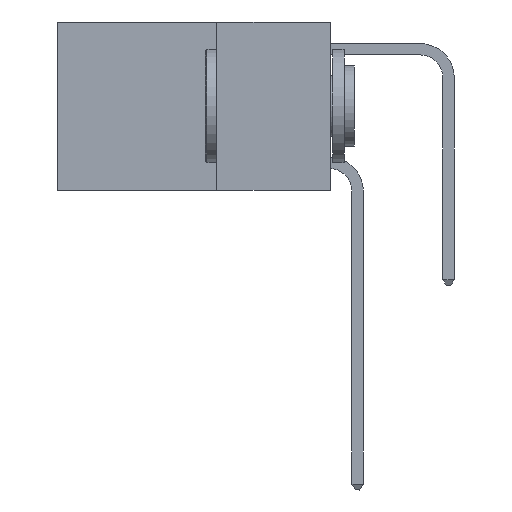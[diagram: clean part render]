
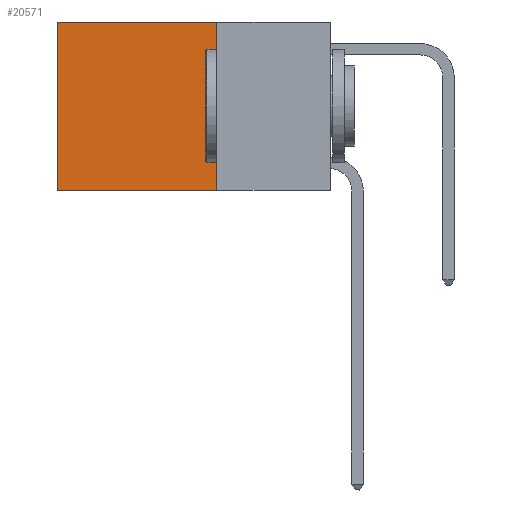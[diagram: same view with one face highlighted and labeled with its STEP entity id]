
A CAD part, left-side view. The second image highlights one B-rep face of the part: STEP entity #20571.
In plain terms, the highlighted planar face has unit normal (-1, 0, 0).
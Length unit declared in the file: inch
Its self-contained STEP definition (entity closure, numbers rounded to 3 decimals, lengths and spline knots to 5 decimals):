
#109 = CARTESIAN_POINT ( 'NONE',  ( 0.2625, 0.25, -0.37 ) ) ;
#2803 = LINE ( 'NONE', #15874, #11579 ) ;
#3349 = LINE ( 'NONE', #4680, #21914 ) ;
#3725 = VERTEX_POINT ( 'NONE', #13115 ) ;
#4546 = FACE_OUTER_BOUND ( 'NONE', #17634, .T. ) ;
#4548 = DIRECTION ( 'NONE',  ( 0., 0., -1. ) ) ;
#4680 = CARTESIAN_POINT ( 'NONE',  ( 0.2625, 0.25, 0. ) ) ;
#6588 = CARTESIAN_POINT ( 'NONE',  ( 0.2625, 0.25, 0. ) ) ;
#6670 = DIRECTION ( 'NONE',  ( 1., 0., 0. ) ) ;
#7106 = DIRECTION ( 'NONE',  ( 0., 1., 0. ) ) ;
#8659 = VECTOR ( 'NONE', #13685, 39.37008 ) ;
#8746 = ORIENTED_EDGE ( 'NONE', *, *, #20583, .T. ) ;
#9796 = VERTEX_POINT ( 'NONE', #109 ) ;
#9812 = EDGE_CURVE ( 'NONE', #9796, #16603, #2803, .T. ) ;
#9827 = CARTESIAN_POINT ( 'NONE',  ( 0.2625, 0.6, 0. ) ) ;
#10000 = VERTEX_POINT ( 'NONE', #21564 ) ;
#10196 = EDGE_CURVE ( 'NONE', #10000, #9796, #3349, .T. ) ;
#10614 = VECTOR ( 'NONE', #4548, 39.37008 ) ;
#10733 = ORIENTED_EDGE ( 'NONE', *, *, #10196, .F. ) ;
#11579 = VECTOR ( 'NONE', #7106, 39.37008 ) ;
#11925 = CARTESIAN_POINT ( 'NONE',  ( 0.2625, 0.25, 0. ) ) ;
#12843 = AXIS2_PLACEMENT_3D ( 'NONE', #6588, #6670, #18924 ) ;
#13115 = CARTESIAN_POINT ( 'NONE',  ( 0.2625, 0.6, 0. ) ) ;
#13685 = DIRECTION ( 'NONE',  ( 0., 1., 0. ) ) ;
#13873 = LINE ( 'NONE', #11925, #8659 ) ;
#14257 = EDGE_CURVE ( 'NONE', #3725, #16603, #19942, .T. ) ;
#15233 = DIRECTION ( 'NONE',  ( 0., 0., -1. ) ) ;
#15874 = CARTESIAN_POINT ( 'NONE',  ( 0.2625, 0.25, -0.37 ) ) ;
#16603 = VERTEX_POINT ( 'NONE', #22393 ) ;
#17150 = PLANE ( 'NONE',  #12843 ) ;
#17634 = EDGE_LOOP ( 'NONE', ( #18019, #20479, #10733, #8746 ) ) ;
#18019 = ORIENTED_EDGE ( 'NONE', *, *, #14257, .T. ) ;
#18924 = DIRECTION ( 'NONE',  ( 0., 0., -1. ) ) ;
#19942 = LINE ( 'NONE', #9827, #10614 ) ;
#20479 = ORIENTED_EDGE ( 'NONE', *, *, #9812, .F. ) ;
#20571 = ADVANCED_FACE ( 'NONE', ( #4546 ), #17150, .F. ) ;
#20583 = EDGE_CURVE ( 'NONE', #10000, #3725, #13873, .T. ) ;
#21564 = CARTESIAN_POINT ( 'NONE',  ( 0.2625, 0.25, 0. ) ) ;
#21914 = VECTOR ( 'NONE', #15233, 39.37008 ) ;
#22393 = CARTESIAN_POINT ( 'NONE',  ( 0.2625, 0.6, -0.37 ) ) ;
